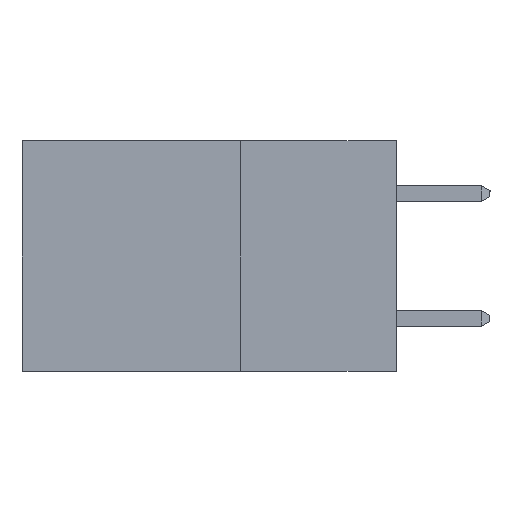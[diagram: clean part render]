
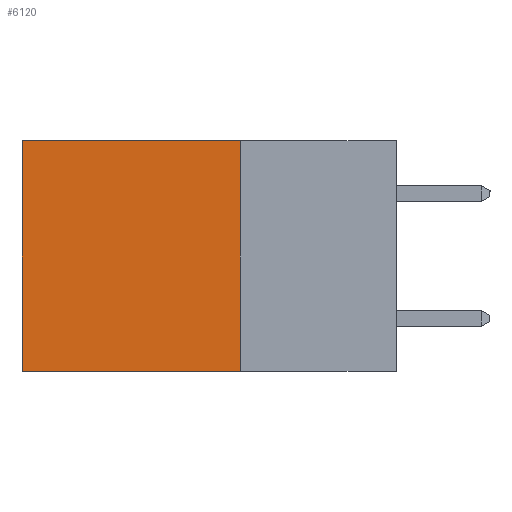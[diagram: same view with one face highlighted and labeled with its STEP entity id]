
A CAD part, left-side view. The second image highlights one B-rep face of the part: STEP entity #6120.
In plain terms, the highlighted planar face has unit normal (-1, 0, 0).
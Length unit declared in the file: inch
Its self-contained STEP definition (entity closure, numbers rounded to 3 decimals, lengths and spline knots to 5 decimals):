
#85 = VERTEX_POINT ( 'NONE', #1677 ) ;
#946 = VECTOR ( 'NONE', #1699, 39.37008 ) ;
#1400 = LINE ( 'NONE', #5143, #13837 ) ;
#1544 = CARTESIAN_POINT ( 'NONE',  ( 0.2615, 0.6, -0.37 ) ) ;
#1677 = CARTESIAN_POINT ( 'NONE',  ( 0.2615, 0.6, 0. ) ) ;
#1699 = DIRECTION ( 'NONE',  ( 0., 0., -1. ) ) ;
#1706 = LINE ( 'NONE', #3212, #3940 ) ;
#2337 = VECTOR ( 'NONE', #12676, 39.37008 ) ;
#2865 = ORIENTED_EDGE ( 'NONE', *, *, #13566, .T. ) ;
#2870 = CARTESIAN_POINT ( 'NONE',  ( 0.2615, 0.6, -0.37 ) ) ;
#3108 = ORIENTED_EDGE ( 'NONE', *, *, #9039, .F. ) ;
#3212 = CARTESIAN_POINT ( 'NONE',  ( 0.2615, 0.25, 0. ) ) ;
#3271 = CARTESIAN_POINT ( 'NONE',  ( 0.2615, 0.25, -0.37 ) ) ;
#3940 = VECTOR ( 'NONE', #11955, 39.37008 ) ;
#4329 = EDGE_CURVE ( 'NONE', #14168, #10373, #14250, .T. ) ;
#5143 = CARTESIAN_POINT ( 'NONE',  ( 0.2615, 0.25, -0.37 ) ) ;
#5272 = DIRECTION ( 'NONE',  ( 0., 0., -1. ) ) ;
#6063 = ORIENTED_EDGE ( 'NONE', *, *, #4329, .F. ) ;
#6120 = ADVANCED_FACE ( 'NONE', ( #8920 ), #10418, .F. ) ;
#7682 = EDGE_LOOP ( 'NONE', ( #2865, #3108, #6063, #14070 ) ) ;
#7741 = DIRECTION ( 'NONE',  ( 1., 0., 0. ) ) ;
#7824 = CARTESIAN_POINT ( 'NONE',  ( 0.2615, 0.25, -0.37 ) ) ;
#8315 = EDGE_CURVE ( 'NONE', #14168, #85, #1706, .T. ) ;
#8920 = FACE_OUTER_BOUND ( 'NONE', #7682, .T. ) ;
#9039 = EDGE_CURVE ( 'NONE', #10373, #14860, #1400, .T. ) ;
#9504 = CARTESIAN_POINT ( 'NONE',  ( 0.2615, 0.25, 0. ) ) ;
#10373 = VERTEX_POINT ( 'NONE', #3271 ) ;
#10418 = PLANE ( 'NONE',  #13050 ) ;
#11955 = DIRECTION ( 'NONE',  ( 0., 1., 0. ) ) ;
#12676 = DIRECTION ( 'NONE',  ( 0., 0., -1. ) ) ;
#13050 = AXIS2_PLACEMENT_3D ( 'NONE', #7824, #7741, #5272 ) ;
#13097 = LINE ( 'NONE', #2870, #946 ) ;
#13566 = EDGE_CURVE ( 'NONE', #85, #14860, #13097, .T. ) ;
#13837 = VECTOR ( 'NONE', #15534, 39.37008 ) ;
#14003 = CARTESIAN_POINT ( 'NONE',  ( 0.2615, 0.25, -0.37 ) ) ;
#14070 = ORIENTED_EDGE ( 'NONE', *, *, #8315, .T. ) ;
#14168 = VERTEX_POINT ( 'NONE', #9504 ) ;
#14250 = LINE ( 'NONE', #14003, #2337 ) ;
#14860 = VERTEX_POINT ( 'NONE', #1544 ) ;
#15534 = DIRECTION ( 'NONE',  ( 0., 1., 0. ) ) ;
